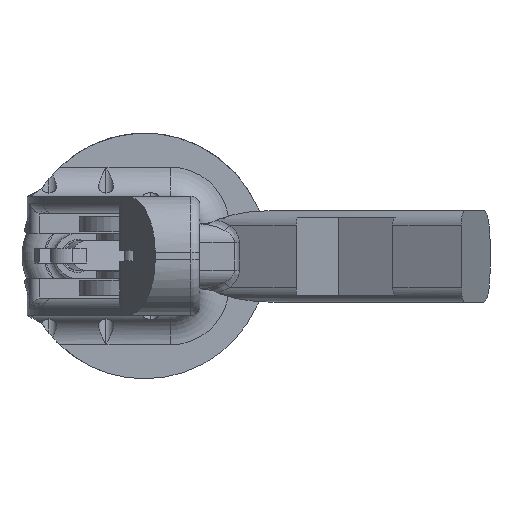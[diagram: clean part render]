
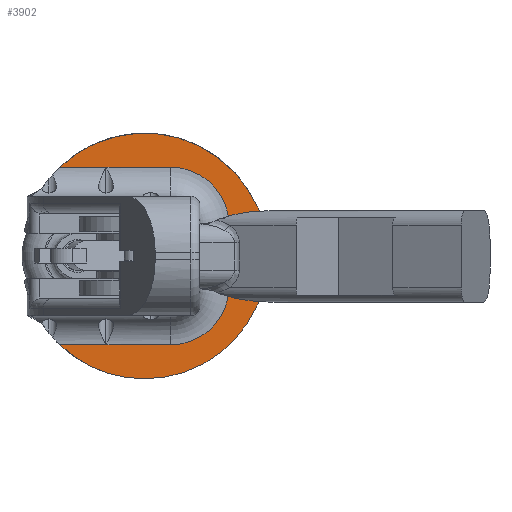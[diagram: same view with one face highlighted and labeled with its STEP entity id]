
A CAD part, left-side view. The second image highlights one B-rep face of the part: STEP entity #3902.
In plain terms, the highlighted planar face has unit normal (-1, 0, 0).
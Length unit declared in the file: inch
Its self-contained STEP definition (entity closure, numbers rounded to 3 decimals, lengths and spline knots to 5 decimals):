
#243 = PLANE ( 'NONE',  #22763 ) ;
#994 = DIRECTION ( 'NONE',  ( 1., 0., 0. ) ) ;
#1232 = CARTESIAN_POINT ( 'NONE',  ( -1.3, 2.31584, -0.3937 ) ) ;
#1297 = CIRCLE ( 'NONE', #2981, 0.7874 ) ;
#1451 = CARTESIAN_POINT ( 'NONE',  ( -1.3, 2.31584, -0.3937 ) ) ;
#1555 = EDGE_LOOP ( 'NONE', ( #11684, #10796, #12823, #11289, #6679, #8042, #10614, #7887, #19985, #10631, #4623, #6666, #5701, #22110, #21210, #9790, #3597 ) ) ;
#1666 = EDGE_CURVE ( 'NONE', #21906, #22131, #19791, .T. ) ;
#2180 = CARTESIAN_POINT ( 'NONE',  ( -1.3, 1.26, -0.3937 ) ) ;
#2203 = CARTESIAN_POINT ( 'NONE',  ( -1.3, -1.08189, 1.23311 ) ) ;
#2356 = DIRECTION ( 'NONE',  ( 0., 1., 0. ) ) ;
#2570 = EDGE_CURVE ( 'NONE', #22131, #11472, #17221, .T. ) ;
#2820 = FACE_OUTER_BOUND ( 'NONE', #1555, .T. ) ;
#2981 = AXIS2_PLACEMENT_3D ( 'NONE', #20685, #9894, #22490 ) ;
#3041 = VERTEX_POINT ( 'NONE', #2203 ) ;
#3313 = VECTOR ( 'NONE', #12339, 39.37008 ) ;
#3597 = ORIENTED_EDGE ( 'NONE', *, *, #12488, .T. ) ;
#3646 = DIRECTION ( 'NONE',  ( 1., 0., 0. ) ) ;
#3790 = CARTESIAN_POINT ( 'NONE',  ( -1.3, 0.74082, 0.8 ) ) ;
#3875 = LINE ( 'NONE', #15964, #3313 ) ;
#3902 = ADVANCED_FACE ( 'NONE', ( #2820 ), #243, .F. ) ;
#3947 = DIRECTION ( 'NONE',  ( 1., 0., 0. ) ) ;
#4623 = ORIENTED_EDGE ( 'NONE', *, *, #9587, .T. ) ;
#5305 = CIRCLE ( 'NONE', #18409, 0.3937 ) ;
#5625 = DIRECTION ( 'NONE',  ( 0., 0., -1. ) ) ;
#5701 = ORIENTED_EDGE ( 'NONE', *, *, #14650, .T. ) ;
#5709 = DIRECTION ( 'NONE',  ( 1., 0., 0. ) ) ;
#5954 = LINE ( 'NONE', #10008, #10281 ) ;
#6135 = EDGE_CURVE ( 'NONE', #12940, #10942, #3875, .T. ) ;
#6407 = VERTEX_POINT ( 'NONE', #11288 ) ;
#6666 = ORIENTED_EDGE ( 'NONE', *, *, #17570, .T. ) ;
#6679 = ORIENTED_EDGE ( 'NONE', *, *, #17687, .T. ) ;
#6715 = CARTESIAN_POINT ( 'NONE',  ( -1.3, 1.87993, 1.9937 ) ) ;
#6795 = VERTEX_POINT ( 'NONE', #17696 ) ;
#7015 = CIRCLE ( 'NONE', #23218, 0.3937 ) ;
#7136 = VECTOR ( 'NONE', #19873, 39.37008 ) ;
#7231 = CARTESIAN_POINT ( 'NONE',  ( -1.3, -1.2, 1.9937 ) ) ;
#7427 = CARTESIAN_POINT ( 'NONE',  ( -1.3, -0.3937, 1.2063 ) ) ;
#7509 = VECTOR ( 'NONE', #2356, 39.37008 ) ;
#7753 = EDGE_CURVE ( 'NONE', #21906, #19811, #5305, .T. ) ;
#7865 = CARTESIAN_POINT ( 'NONE',  ( -1.3, 0.3937, 1.9937 ) ) ;
#7887 = ORIENTED_EDGE ( 'NONE', *, *, #1666, .F. ) ;
#8031 = LINE ( 'NONE', #13624, #15413 ) ;
#8042 = ORIENTED_EDGE ( 'NONE', *, *, #10625, .T. ) ;
#8683 = VERTEX_POINT ( 'NONE', #17170 ) ;
#8978 = VERTEX_POINT ( 'NONE', #7427 ) ;
#9090 = AXIS2_PLACEMENT_3D ( 'NONE', #3790, #16487, #5625 ) ;
#9350 = LINE ( 'NONE', #9771, #13606 ) ;
#9411 = DIRECTION ( 'NONE',  ( 1., 0., 0. ) ) ;
#9587 = EDGE_CURVE ( 'NONE', #12022, #11254, #21354, .T. ) ;
#9771 = CARTESIAN_POINT ( 'NONE',  ( -1.3, -1.2, 1.23311 ) ) ;
#9790 = ORIENTED_EDGE ( 'NONE', *, *, #21553, .F. ) ;
#9894 = DIRECTION ( 'NONE',  ( 1., 0., 0. ) ) ;
#10008 = CARTESIAN_POINT ( 'NONE',  ( -1.3, -0.51102, 1.115 ) ) ;
#10281 = VECTOR ( 'NONE', #17164, 39.37008 ) ;
#10498 = EDGE_CURVE ( 'NONE', #3041, #17436, #8031, .T. ) ;
#10614 = ORIENTED_EDGE ( 'NONE', *, *, #2570, .F. ) ;
#10625 = EDGE_CURVE ( 'NONE', #15788, #11472, #17365, .T. ) ;
#10631 = ORIENTED_EDGE ( 'NONE', *, *, #12217, .T. ) ;
#10731 = CARTESIAN_POINT ( 'NONE',  ( -1.3, 1.26, 1.9937 ) ) ;
#10768 = CARTESIAN_POINT ( 'NONE',  ( -1.3, 0.3937, 0.3937 ) ) ;
#10796 = ORIENTED_EDGE ( 'NONE', *, *, #22527, .T. ) ;
#10942 = VERTEX_POINT ( 'NONE', #7865 ) ;
#11136 = CARTESIAN_POINT ( 'NONE',  ( -1.3, -1.2, 0.36 ) ) ;
#11254 = VERTEX_POINT ( 'NONE', #13305 ) ;
#11288 = CARTESIAN_POINT ( 'NONE',  ( -1.3, -0.76565, 1.4731 ) ) ;
#11289 = ORIENTED_EDGE ( 'NONE', *, *, #12077, .T. ) ;
#11385 = LINE ( 'NONE', #7231, #7136 ) ;
#11472 = VERTEX_POINT ( 'NONE', #21098 ) ;
#11505 = VERTEX_POINT ( 'NONE', #6715 ) ;
#11655 = VECTOR ( 'NONE', #12139, 39.37008 ) ;
#11684 = ORIENTED_EDGE ( 'NONE', *, *, #6135, .T. ) ;
#11909 = CARTESIAN_POINT ( 'NONE',  ( -1.3, -1.1251, 1.6337 ) ) ;
#12022 = VERTEX_POINT ( 'NONE', #17686 ) ;
#12077 = EDGE_CURVE ( 'NONE', #6795, #8683, #14508, .T. ) ;
#12139 = DIRECTION ( 'NONE',  ( 0., 1., 0. ) ) ;
#12217 = EDGE_CURVE ( 'NONE', #19811, #12022, #21838, .T. ) ;
#12339 = DIRECTION ( 'NONE',  ( 0., -1., 0. ) ) ;
#12428 = CIRCLE ( 'NONE', #13308, 1.65 ) ;
#12488 = EDGE_CURVE ( 'NONE', #11505, #12940, #11385, .T. ) ;
#12562 = DIRECTION ( 'NONE',  ( 0., 1., 0. ) ) ;
#12585 = AXIS2_PLACEMENT_3D ( 'NONE', #14809, #3947, #16630 ) ;
#12823 = ORIENTED_EDGE ( 'NONE', *, *, #16971, .T. ) ;
#12940 = VERTEX_POINT ( 'NONE', #10731 ) ;
#13305 = CARTESIAN_POINT ( 'NONE',  ( -1.3, -0.51102, 0.36689 ) ) ;
#13308 = AXIS2_PLACEMENT_3D ( 'NONE', #14518, #3646, #16335 ) ;
#13606 = VECTOR ( 'NONE', #22302, 39.37008 ) ;
#13624 = CARTESIAN_POINT ( 'NONE',  ( -1.3, -1.08189, 0.36 ) ) ;
#13702 = DIRECTION ( 'NONE',  ( 0., 1., 0. ) ) ;
#14150 = DIRECTION ( 'NONE',  ( 0., 1., 0. ) ) ;
#14508 = CIRCLE ( 'NONE', #20921, 0.7874 ) ;
#14518 = CARTESIAN_POINT ( 'NONE',  ( -1.3, 0.74082, 0.8 ) ) ;
#14650 = EDGE_CURVE ( 'NONE', #15543, #3041, #9350, .T. ) ;
#14809 = CARTESIAN_POINT ( 'NONE',  ( -1.3, 0.74082, 0.8 ) ) ;
#14887 = VECTOR ( 'NONE', #16894, 39.37008 ) ;
#15063 = CARTESIAN_POINT ( 'NONE',  ( -1.3, -0.51102, 0.36689 ) ) ;
#15413 = VECTOR ( 'NONE', #17321, 39.37008 ) ;
#15543 = VERTEX_POINT ( 'NONE', #21276 ) ;
#15788 = VERTEX_POINT ( 'NONE', #2180 ) ;
#15958 = EDGE_CURVE ( 'NONE', #17436, #6407, #7015, .T. ) ;
#15964 = CARTESIAN_POINT ( 'NONE',  ( -1.3, -1.2, 1.9937 ) ) ;
#16335 = DIRECTION ( 'NONE',  ( 0., 0., -1. ) ) ;
#16344 = DIRECTION ( 'NONE',  ( 0., 0., 1. ) ) ;
#16487 = DIRECTION ( 'NONE',  ( 1., 0., 0. ) ) ;
#16630 = DIRECTION ( 'NONE',  ( 0., 0., -1. ) ) ;
#16769 = CARTESIAN_POINT ( 'NONE',  ( -1.3, -1.08189, 1.24238 ) ) ;
#16894 = DIRECTION ( 'NONE',  ( 0., 0., -1. ) ) ;
#16971 = EDGE_CURVE ( 'NONE', #8978, #6795, #19688, .T. ) ;
#17164 = DIRECTION ( 'NONE',  ( 0., 0., 1. ) ) ;
#17170 = CARTESIAN_POINT ( 'NONE',  ( -1.3, 0.3937, -0.3937 ) ) ;
#17221 = CIRCLE ( 'NONE', #12585, 1.65 ) ;
#17321 = DIRECTION ( 'NONE',  ( 0., 0., 1. ) ) ;
#17365 = LINE ( 'NONE', #1451, #22151 ) ;
#17436 = VERTEX_POINT ( 'NONE', #16769 ) ;
#17570 = EDGE_CURVE ( 'NONE', #11254, #15543, #5954, .T. ) ;
#17686 = CARTESIAN_POINT ( 'NONE',  ( -1.3, -1.08189, 0.36689 ) ) ;
#17687 = EDGE_CURVE ( 'NONE', #8683, #15788, #21247, .T. ) ;
#17696 = CARTESIAN_POINT ( 'NONE',  ( -1.3, -0.3937, 0.3937 ) ) ;
#18379 = DIRECTION ( 'NONE',  ( 0., 1., 0. ) ) ;
#18392 = CARTESIAN_POINT ( 'NONE',  ( -1.3, -1.08189, 0.35762 ) ) ;
#18409 = AXIS2_PLACEMENT_3D ( 'NONE', #20212, #9411, #22034 ) ;
#19688 = LINE ( 'NONE', #20376, #14887 ) ;
#19791 = CIRCLE ( 'NONE', #9090, 1.65 ) ;
#19811 = VERTEX_POINT ( 'NONE', #18392 ) ;
#19873 = DIRECTION ( 'NONE',  ( 0., -1., 0. ) ) ;
#19985 = ORIENTED_EDGE ( 'NONE', *, *, #7753, .T. ) ;
#20079 = CARTESIAN_POINT ( 'NONE',  ( -1.3, -0.76565, 0.1269 ) ) ;
#20212 = CARTESIAN_POINT ( 'NONE',  ( -1.3, -1.1251, -0.0337 ) ) ;
#20376 = CARTESIAN_POINT ( 'NONE',  ( -1.3, -0.3937, 0. ) ) ;
#20685 = CARTESIAN_POINT ( 'NONE',  ( -1.3, 0.3937, 1.2063 ) ) ;
#20921 = AXIS2_PLACEMENT_3D ( 'NONE', #10768, #23371, #12562 ) ;
#21098 = CARTESIAN_POINT ( 'NONE',  ( -1.3, 1.87993, -0.3937 ) ) ;
#21210 = ORIENTED_EDGE ( 'NONE', *, *, #15958, .T. ) ;
#21247 = LINE ( 'NONE', #1232, #11655 ) ;
#21275 = VECTOR ( 'NONE', #16344, 39.37008 ) ;
#21276 = CARTESIAN_POINT ( 'NONE',  ( -1.3, -0.51102, 1.23311 ) ) ;
#21354 = LINE ( 'NONE', #15063, #7509 ) ;
#21553 = EDGE_CURVE ( 'NONE', #11505, #6407, #12428, .T. ) ;
#21781 = CARTESIAN_POINT ( 'NONE',  ( -1.3, -1.08189, 0.36 ) ) ;
#21838 = LINE ( 'NONE', #21781, #21275 ) ;
#21906 = VERTEX_POINT ( 'NONE', #20079 ) ;
#22034 = DIRECTION ( 'NONE',  ( 0., 1., 0. ) ) ;
#22110 = ORIENTED_EDGE ( 'NONE', *, *, #10498, .T. ) ;
#22131 = VERTEX_POINT ( 'NONE', #22945 ) ;
#22151 = VECTOR ( 'NONE', #14150, 39.37008 ) ;
#22302 = DIRECTION ( 'NONE',  ( 0., -1., 0. ) ) ;
#22490 = DIRECTION ( 'NONE',  ( 0., 1., 0. ) ) ;
#22527 = EDGE_CURVE ( 'NONE', #10942, #8978, #1297, .T. ) ;
#22763 = AXIS2_PLACEMENT_3D ( 'NONE', #11136, #5709, #18379 ) ;
#22945 = CARTESIAN_POINT ( 'NONE',  ( -1.3, 0.74082, -0.85 ) ) ;
#23218 = AXIS2_PLACEMENT_3D ( 'NONE', #11909, #994, #13702 ) ;
#23371 = DIRECTION ( 'NONE',  ( 1., 0., 0. ) ) ;
